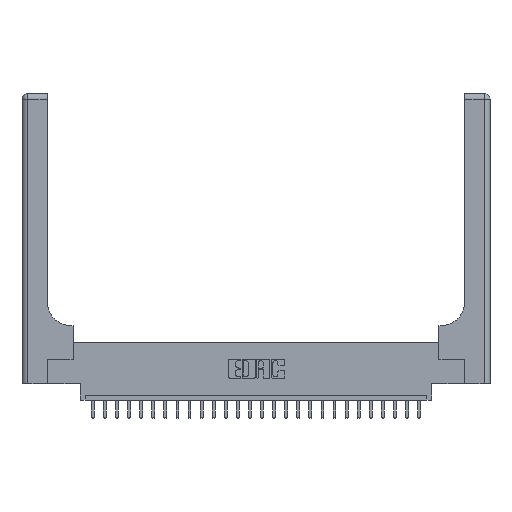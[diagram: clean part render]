
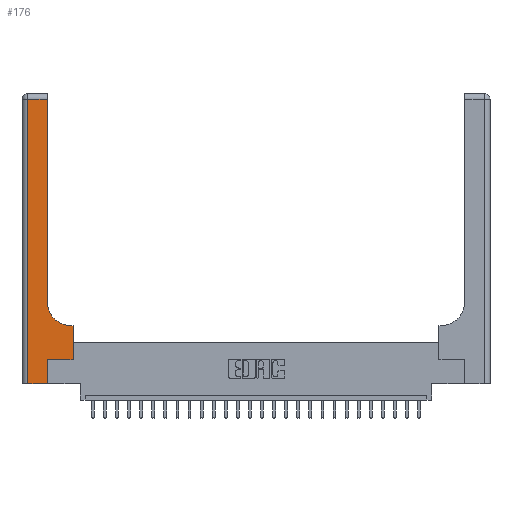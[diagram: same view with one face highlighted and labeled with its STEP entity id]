
A CAD part, top view. The second image highlights one B-rep face of the part: STEP entity #176.
In plain terms, the highlighted planar face has unit normal (0, 0, 1).
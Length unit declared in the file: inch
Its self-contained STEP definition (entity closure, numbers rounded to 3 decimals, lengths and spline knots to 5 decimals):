
#37 = CARTESIAN_POINT ( 'NONE',  ( 0.26, 0.85, 0.37 ) ) ;
#176 = ADVANCED_FACE ( 'NONE', ( #5088 ), #6746, .F. ) ;
#321 = ORIENTED_EDGE ( 'NONE', *, *, #6625, .T. ) ;
#356 = DIRECTION ( 'NONE',  ( -1., 0., 0. ) ) ;
#555 = LINE ( 'NONE', #8310, #4516 ) ;
#917 = DIRECTION ( 'NONE',  ( 0., 1., 0. ) ) ;
#1043 = CARTESIAN_POINT ( 'NONE',  ( 0.06, 2.94, 0.37 ) ) ;
#2024 = CARTESIAN_POINT ( 'NONE',  ( 0.528, 0.25, 0.37 ) ) ;
#2179 = DIRECTION ( 'NONE',  ( 0., -1., 0. ) ) ;
#2317 = CARTESIAN_POINT ( 'NONE',  ( 0.265, 0., 0.37 ) ) ;
#3280 = LINE ( 'NONE', #11044, #17732 ) ;
#3664 = VERTEX_POINT ( 'NONE', #15836 ) ;
#3833 = LINE ( 'NONE', #4199, #18251 ) ;
#3851 = VERTEX_POINT ( 'NONE', #37 ) ;
#4062 = VERTEX_POINT ( 'NONE', #2317 ) ;
#4199 = CARTESIAN_POINT ( 'NONE',  ( 0.06, 3., 0.37 ) ) ;
#4368 = EDGE_LOOP ( 'NONE', ( #321, #8016, #20442, #16798, #13301, #11550, #16493, #7787, #23263 ) ) ;
#4516 = VECTOR ( 'NONE', #4869, 39.37008 ) ;
#4869 = DIRECTION ( 'NONE',  ( -1., 0., 0. ) ) ;
#5001 = DIRECTION ( 'NONE',  ( 1., 0., 0. ) ) ;
#5088 = FACE_OUTER_BOUND ( 'NONE', #4368, .T. ) ;
#5400 = VECTOR ( 'NONE', #5001, 39.37008 ) ;
#6065 = CARTESIAN_POINT ( 'NONE',  ( 0.265, 0., 0.37 ) ) ;
#6159 = LINE ( 'NONE', #23465, #5400 ) ;
#6322 = CARTESIAN_POINT ( 'NONE',  ( 0.26, 0.6, 0.37 ) ) ;
#6625 = EDGE_CURVE ( 'NONE', #3851, #24072, #12119, .T. ) ;
#6729 = AXIS2_PLACEMENT_3D ( 'NONE', #9030, #20471, #24423 ) ;
#6746 = PLANE ( 'NONE',  #6729 ) ;
#7670 = EDGE_CURVE ( 'NONE', #24893, #25086, #3280, .T. ) ;
#7787 = ORIENTED_EDGE ( 'NONE', *, *, #8898, .T. ) ;
#8016 = ORIENTED_EDGE ( 'NONE', *, *, #15600, .T. ) ;
#8294 = AXIS2_PLACEMENT_3D ( 'NONE', #10051, #13966, #12069 ) ;
#8310 = CARTESIAN_POINT ( 'NONE',  ( 0., 2.94, 0.37 ) ) ;
#8694 = DIRECTION ( 'NONE',  ( 0., 1., 0. ) ) ;
#8855 = VERTEX_POINT ( 'NONE', #21948 ) ;
#8898 = EDGE_CURVE ( 'NONE', #24180, #8855, #10259, .T. ) ;
#9030 = CARTESIAN_POINT ( 'NONE',  ( 0., 3., 0.37 ) ) ;
#10051 = CARTESIAN_POINT ( 'NONE',  ( 0.51, 0.85, 0.37 ) ) ;
#10259 = LINE ( 'NONE', #6322, #15723 ) ;
#11044 = CARTESIAN_POINT ( 'NONE',  ( 0.265, 0.25, 0.37 ) ) ;
#11550 = ORIENTED_EDGE ( 'NONE', *, *, #7670, .T. ) ;
#11712 = EDGE_CURVE ( 'NONE', #16070, #3664, #3833, .T. ) ;
#11897 = VECTOR ( 'NONE', #8694, 39.37008 ) ;
#12069 = DIRECTION ( 'NONE',  ( 1., 0., 0. ) ) ;
#12119 = LINE ( 'NONE', #12244, #11897 ) ;
#12244 = CARTESIAN_POINT ( 'NONE',  ( 0.26, 3., 0.37 ) ) ;
#12353 = EDGE_CURVE ( 'NONE', #4062, #24893, #21451, .T. ) ;
#13301 = ORIENTED_EDGE ( 'NONE', *, *, #12353, .T. ) ;
#13966 = DIRECTION ( 'NONE',  ( 0., 0., -1. ) ) ;
#14967 = DIRECTION ( 'NONE',  ( 1., 0., 0. ) ) ;
#15600 = EDGE_CURVE ( 'NONE', #24072, #16070, #555, .T. ) ;
#15723 = VECTOR ( 'NONE', #356, 39.37008 ) ;
#15836 = CARTESIAN_POINT ( 'NONE',  ( 0.06, 0., 0.37 ) ) ;
#15988 = CIRCLE ( 'NONE', #8294, 0.25 ) ;
#16070 = VERTEX_POINT ( 'NONE', #1043 ) ;
#16161 = LINE ( 'NONE', #23934, #17216 ) ;
#16479 = CARTESIAN_POINT ( 'NONE',  ( 0.26, 2.94, 0.37 ) ) ;
#16493 = ORIENTED_EDGE ( 'NONE', *, *, #22016, .T. ) ;
#16798 = ORIENTED_EDGE ( 'NONE', *, *, #16821, .T. ) ;
#16821 = EDGE_CURVE ( 'NONE', #3664, #4062, #6159, .T. ) ;
#17216 = VECTOR ( 'NONE', #917, 39.37008 ) ;
#17732 = VECTOR ( 'NONE', #14967, 39.37008 ) ;
#18251 = VECTOR ( 'NONE', #2179, 39.37008 ) ;
#20305 = VECTOR ( 'NONE', #21202, 39.37008 ) ;
#20442 = ORIENTED_EDGE ( 'NONE', *, *, #11712, .T. ) ;
#20471 = DIRECTION ( 'NONE',  ( 0., 0., -1. ) ) ;
#21202 = DIRECTION ( 'NONE',  ( 0., 1., 0. ) ) ;
#21451 = LINE ( 'NONE', #6065, #20305 ) ;
#21647 = CARTESIAN_POINT ( 'NONE',  ( 0.528, 0.6, 0.37 ) ) ;
#21948 = CARTESIAN_POINT ( 'NONE',  ( 0.51, 0.6, 0.37 ) ) ;
#22016 = EDGE_CURVE ( 'NONE', #25086, #24180, #16161, .T. ) ;
#22369 = CARTESIAN_POINT ( 'NONE',  ( 0.265, 0.25, 0.37 ) ) ;
#23263 = ORIENTED_EDGE ( 'NONE', *, *, #23574, .T. ) ;
#23465 = CARTESIAN_POINT ( 'NONE',  ( 0., 0., 0.37 ) ) ;
#23574 = EDGE_CURVE ( 'NONE', #8855, #3851, #15988, .T. ) ;
#23934 = CARTESIAN_POINT ( 'NONE',  ( 0.528, 0.25, 0.37 ) ) ;
#24072 = VERTEX_POINT ( 'NONE', #16479 ) ;
#24180 = VERTEX_POINT ( 'NONE', #21647 ) ;
#24423 = DIRECTION ( 'NONE',  ( -1., 0., 0. ) ) ;
#24893 = VERTEX_POINT ( 'NONE', #22369 ) ;
#25086 = VERTEX_POINT ( 'NONE', #2024 ) ;
